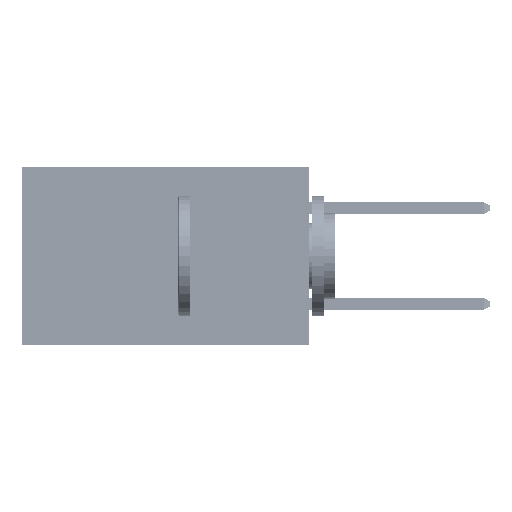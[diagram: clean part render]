
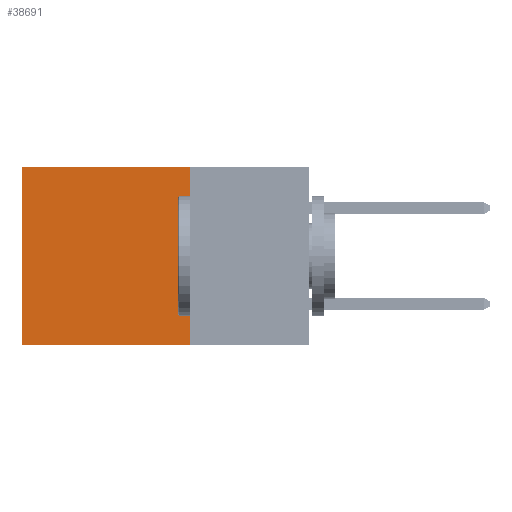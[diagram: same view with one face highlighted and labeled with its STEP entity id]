
A CAD part, left-side view. The second image highlights one B-rep face of the part: STEP entity #38691.
In plain terms, the highlighted planar face has unit normal (-1, 0, 0).
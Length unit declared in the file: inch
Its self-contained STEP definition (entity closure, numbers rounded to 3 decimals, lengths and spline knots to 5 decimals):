
#347 = DIRECTION ( 'NONE',  ( 0., 0., -1. ) ) ;
#1064 = FACE_OUTER_BOUND ( 'NONE', #31983, .T. ) ;
#5401 = PLANE ( 'NONE',  #16786 ) ;
#5638 = VECTOR ( 'NONE', #47161, 39.37008 ) ;
#6593 = CARTESIAN_POINT ( 'NONE',  ( 0.2875, 0.25, -0.37 ) ) ;
#7900 = CARTESIAN_POINT ( 'NONE',  ( 0.2875, 0.6, 0. ) ) ;
#10528 = VERTEX_POINT ( 'NONE', #27566 ) ;
#12266 = LINE ( 'NONE', #7900, #28756 ) ;
#12376 = CARTESIAN_POINT ( 'NONE',  ( 0.2875, 0.25, 0. ) ) ;
#14627 = EDGE_CURVE ( 'NONE', #26470, #29177, #40472, .T. ) ;
#16269 = LINE ( 'NONE', #33253, #49179 ) ;
#16786 = AXIS2_PLACEMENT_3D ( 'NONE', #40408, #28151, #32734 ) ;
#18266 = VERTEX_POINT ( 'NONE', #21942 ) ;
#21942 = CARTESIAN_POINT ( 'NONE',  ( 0.2875, 0.6, 0. ) ) ;
#23062 = ORIENTED_EDGE ( 'NONE', *, *, #14627, .F. ) ;
#23139 = ORIENTED_EDGE ( 'NONE', *, *, #39881, .F. ) ;
#24264 = CARTESIAN_POINT ( 'NONE',  ( 0.2875, 0.6, -0.37 ) ) ;
#26470 = VERTEX_POINT ( 'NONE', #6593 ) ;
#27080 = VECTOR ( 'NONE', #32123, 39.37008 ) ;
#27432 = EDGE_CURVE ( 'NONE', #18266, #29177, #12266, .T. ) ;
#27566 = CARTESIAN_POINT ( 'NONE',  ( 0.2875, 0.25, 0. ) ) ;
#28151 = DIRECTION ( 'NONE',  ( 1., 0., 0. ) ) ;
#28756 = VECTOR ( 'NONE', #347, 39.37008 ) ;
#29177 = VERTEX_POINT ( 'NONE', #24264 ) ;
#29845 = DIRECTION ( 'NONE',  ( 0., 0., -1. ) ) ;
#31983 = EDGE_LOOP ( 'NONE', ( #42636, #23062, #23139, #38724 ) ) ;
#32123 = DIRECTION ( 'NONE',  ( 0., 1., 0. ) ) ;
#32734 = DIRECTION ( 'NONE',  ( 0., 0., -1. ) ) ;
#33253 = CARTESIAN_POINT ( 'NONE',  ( 0.2875, 0.25, 0. ) ) ;
#38691 = ADVANCED_FACE ( 'NONE', ( #1064 ), #5401, .F. ) ;
#38724 = ORIENTED_EDGE ( 'NONE', *, *, #48852, .T. ) ;
#38767 = CARTESIAN_POINT ( 'NONE',  ( 0.2875, 0.25, -0.37 ) ) ;
#39881 = EDGE_CURVE ( 'NONE', #10528, #26470, #16269, .T. ) ;
#40408 = CARTESIAN_POINT ( 'NONE',  ( 0.2875, 0.25, 0. ) ) ;
#40472 = LINE ( 'NONE', #38767, #27080 ) ;
#42636 = ORIENTED_EDGE ( 'NONE', *, *, #27432, .T. ) ;
#47161 = DIRECTION ( 'NONE',  ( 0., 1., 0. ) ) ;
#47828 = LINE ( 'NONE', #12376, #5638 ) ;
#48852 = EDGE_CURVE ( 'NONE', #10528, #18266, #47828, .T. ) ;
#49179 = VECTOR ( 'NONE', #29845, 39.37008 ) ;
